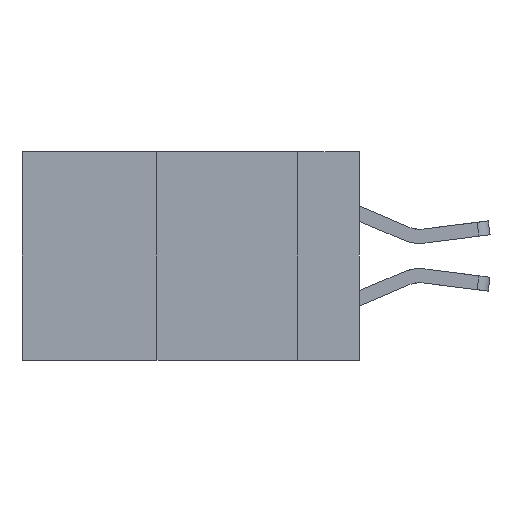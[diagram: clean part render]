
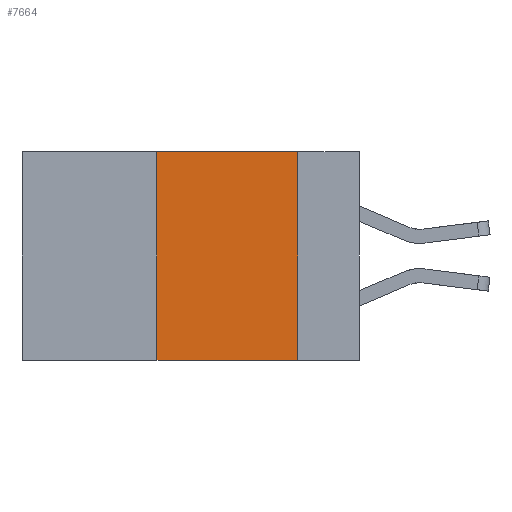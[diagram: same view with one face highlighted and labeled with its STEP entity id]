
A CAD part, left-side view. The second image highlights one B-rep face of the part: STEP entity #7664.
In plain terms, the highlighted planar face has unit normal (-1, 0, 0).
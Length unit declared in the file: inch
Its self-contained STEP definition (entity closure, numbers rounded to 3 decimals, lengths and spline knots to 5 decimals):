
#306 = VECTOR ( 'NONE', #9033, 39.37008 ) ;
#389 = DIRECTION ( 'NONE',  ( 0., 0., 1. ) ) ;
#448 = CARTESIAN_POINT ( 'NONE',  ( 0., 0.36, 0. ) ) ;
#468 = DIRECTION ( 'NONE',  ( 1., 0., 0. ) ) ;
#1224 = CARTESIAN_POINT ( 'NONE',  ( 0., 0.11, 0. ) ) ;
#1535 = CARTESIAN_POINT ( 'NONE',  ( 0., 0.6, -0.37 ) ) ;
#2029 = VERTEX_POINT ( 'NONE', #12823 ) ;
#2228 = LINE ( 'NONE', #3085, #6169 ) ;
#2882 = ORIENTED_EDGE ( 'NONE', *, *, #10255, .F. ) ;
#3016 = DIRECTION ( 'NONE',  ( 0., -1., 0. ) ) ;
#3085 = CARTESIAN_POINT ( 'NONE',  ( 0., 0.6, 0. ) ) ;
#3486 = ORIENTED_EDGE ( 'NONE', *, *, #6530, .F. ) ;
#4159 = CARTESIAN_POINT ( 'NONE',  ( 0., 0.11, 0. ) ) ;
#4482 = LINE ( 'NONE', #448, #8989 ) ;
#4797 = LINE ( 'NONE', #1535, #306 ) ;
#4908 = FACE_OUTER_BOUND ( 'NONE', #8956, .T. ) ;
#5168 = VERTEX_POINT ( 'NONE', #6441 ) ;
#6169 = VECTOR ( 'NONE', #3016, 39.37008 ) ;
#6232 = EDGE_CURVE ( 'NONE', #2029, #5168, #4482, .T. ) ;
#6441 = CARTESIAN_POINT ( 'NONE',  ( 0., 0.36, 0. ) ) ;
#6530 = EDGE_CURVE ( 'NONE', #5168, #6960, #2228, .T. ) ;
#6960 = VERTEX_POINT ( 'NONE', #4159 ) ;
#7664 = ADVANCED_FACE ( 'NONE', ( #4908 ), #8870, .F. ) ;
#7816 = CARTESIAN_POINT ( 'NONE',  ( 0., 0.6, 0. ) ) ;
#8507 = VERTEX_POINT ( 'NONE', #12357 ) ;
#8870 = PLANE ( 'NONE',  #9553 ) ;
#8956 = EDGE_LOOP ( 'NONE', ( #2882, #3486, #12349, #12530 ) ) ;
#8989 = VECTOR ( 'NONE', #389, 39.37008 ) ;
#9033 = DIRECTION ( 'NONE',  ( 0., -1., 0. ) ) ;
#9553 = AXIS2_PLACEMENT_3D ( 'NONE', #7816, #468, #12273 ) ;
#9693 = DIRECTION ( 'NONE',  ( 0., 0., -1. ) ) ;
#10255 = EDGE_CURVE ( 'NONE', #6960, #8507, #12868, .T. ) ;
#11121 = VECTOR ( 'NONE', #9693, 39.37008 ) ;
#12273 = DIRECTION ( 'NONE',  ( 0., 0., -1. ) ) ;
#12349 = ORIENTED_EDGE ( 'NONE', *, *, #6232, .F. ) ;
#12357 = CARTESIAN_POINT ( 'NONE',  ( 0., 0.11, -0.37 ) ) ;
#12530 = ORIENTED_EDGE ( 'NONE', *, *, #12686, .T. ) ;
#12686 = EDGE_CURVE ( 'NONE', #2029, #8507, #4797, .T. ) ;
#12823 = CARTESIAN_POINT ( 'NONE',  ( 0., 0.36, -0.37 ) ) ;
#12868 = LINE ( 'NONE', #1224, #11121 ) ;
